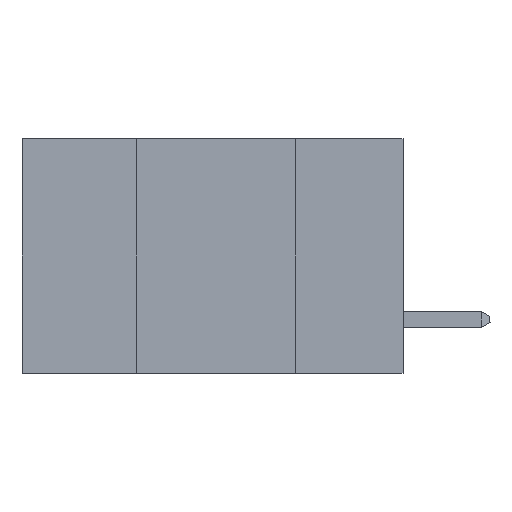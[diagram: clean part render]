
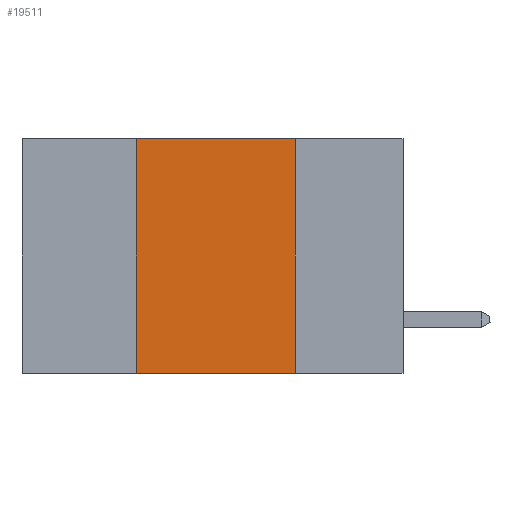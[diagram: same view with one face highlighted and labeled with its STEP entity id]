
A CAD part, left-side view. The second image highlights one B-rep face of the part: STEP entity #19511.
In plain terms, the highlighted planar face has unit normal (-1, 0, 0).
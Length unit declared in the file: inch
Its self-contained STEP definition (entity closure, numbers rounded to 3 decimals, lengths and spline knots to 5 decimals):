
#431 = DIRECTION ( 'NONE',  ( 1., 0., 0. ) ) ;
#661 = CARTESIAN_POINT ( 'NONE',  ( 0., 0.17, 0. ) ) ;
#2044 = CARTESIAN_POINT ( 'NONE',  ( 0., 0.6, 0. ) ) ;
#2826 = CARTESIAN_POINT ( 'NONE',  ( 0., 0.42, -0.37 ) ) ;
#3363 = VECTOR ( 'NONE', #27149, 39.37008 ) ;
#6447 = CARTESIAN_POINT ( 'NONE',  ( 0., 0.42, 0. ) ) ;
#7864 = EDGE_CURVE ( 'NONE', #18545, #30115, #26003, .T. ) ;
#9215 = DIRECTION ( 'NONE',  ( 0., 0., 1. ) ) ;
#9710 = EDGE_CURVE ( 'NONE', #10064, #34979, #19848, .T. ) ;
#10064 = VERTEX_POINT ( 'NONE', #32899 ) ;
#10741 = CARTESIAN_POINT ( 'NONE',  ( 0., 0.17, -0.37 ) ) ;
#11092 = VECTOR ( 'NONE', #19696, 39.37008 ) ;
#12381 = VECTOR ( 'NONE', #17440, 39.37008 ) ;
#14010 = EDGE_LOOP ( 'NONE', ( #33350, #33103, #28473, #31016 ) ) ;
#14062 = CARTESIAN_POINT ( 'NONE',  ( 0., 0.6, -0.37 ) ) ;
#14400 = PLANE ( 'NONE',  #32088 ) ;
#17233 = EDGE_CURVE ( 'NONE', #18545, #34979, #20310, .T. ) ;
#17440 = DIRECTION ( 'NONE',  ( 0., 0., -1. ) ) ;
#18253 = LINE ( 'NONE', #2044, #3363 ) ;
#18545 = VERTEX_POINT ( 'NONE', #2826 ) ;
#19511 = ADVANCED_FACE ( 'NONE', ( #22285 ), #14400, .F. ) ;
#19526 = VECTOR ( 'NONE', #9215, 39.37008 ) ;
#19696 = DIRECTION ( 'NONE',  ( 0., -1., 0. ) ) ;
#19848 = LINE ( 'NONE', #661, #12381 ) ;
#20014 = DIRECTION ( 'NONE',  ( 0., 0., -1. ) ) ;
#20310 = LINE ( 'NONE', #14062, #11092 ) ;
#22285 = FACE_OUTER_BOUND ( 'NONE', #14010, .T. ) ;
#26003 = LINE ( 'NONE', #6447, #19526 ) ;
#27149 = DIRECTION ( 'NONE',  ( 0., -1., 0. ) ) ;
#28473 = ORIENTED_EDGE ( 'NONE', *, *, #7864, .F. ) ;
#29956 = EDGE_CURVE ( 'NONE', #30115, #10064, #18253, .T. ) ;
#30115 = VERTEX_POINT ( 'NONE', #30667 ) ;
#30667 = CARTESIAN_POINT ( 'NONE',  ( 0., 0.42, 0. ) ) ;
#31016 = ORIENTED_EDGE ( 'NONE', *, *, #17233, .T. ) ;
#32088 = AXIS2_PLACEMENT_3D ( 'NONE', #33812, #431, #20014 ) ;
#32899 = CARTESIAN_POINT ( 'NONE',  ( 0., 0.17, 0. ) ) ;
#33103 = ORIENTED_EDGE ( 'NONE', *, *, #29956, .F. ) ;
#33350 = ORIENTED_EDGE ( 'NONE', *, *, #9710, .F. ) ;
#33812 = CARTESIAN_POINT ( 'NONE',  ( 0., 0.6, 0. ) ) ;
#34979 = VERTEX_POINT ( 'NONE', #10741 ) ;
